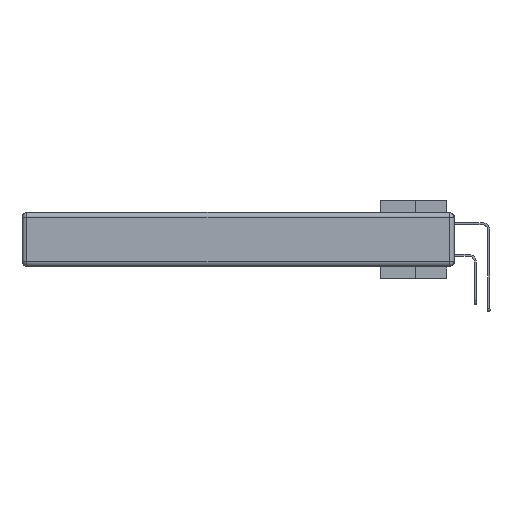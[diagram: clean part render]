
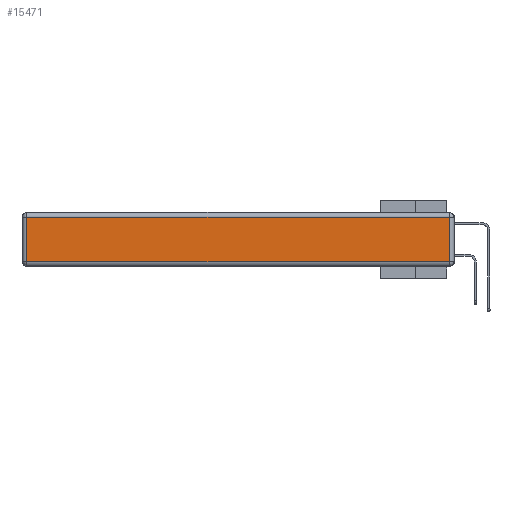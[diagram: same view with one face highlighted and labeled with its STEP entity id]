
A CAD part, left-side view. The second image highlights one B-rep face of the part: STEP entity #15471.
In plain terms, the highlighted planar face has unit normal (-1, 0, 0).
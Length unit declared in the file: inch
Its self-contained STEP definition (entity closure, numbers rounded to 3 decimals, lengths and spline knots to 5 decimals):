
#2451 = ORIENTED_EDGE ( 'NONE', *, *, #8380, .T. ) ;
#2903 = CARTESIAN_POINT ( 'NONE',  ( 0., 0., -0.313 ) ) ;
#3422 = VECTOR ( 'NONE', #16219, 39.37008 ) ;
#3586 = DIRECTION ( 'NONE',  ( 0., 0., -1. ) ) ;
#3810 = CARTESIAN_POINT ( 'NONE',  ( 0., 0., -0.343 ) ) ;
#4682 = VECTOR ( 'NONE', #9215, 39.37008 ) ;
#7297 = CARTESIAN_POINT ( 'NONE',  ( 0., 2.72, -0.343 ) ) ;
#7504 = CARTESIAN_POINT ( 'NONE',  ( 0., 0.03, -0.343 ) ) ;
#7738 = DIRECTION ( 'NONE',  ( 0., 0., 1. ) ) ;
#8380 = EDGE_CURVE ( 'NONE', #20937, #24700, #33931, .T. ) ;
#9215 = DIRECTION ( 'NONE',  ( 0., 1., 0. ) ) ;
#11574 = AXIS2_PLACEMENT_3D ( 'NONE', #3810, #40262, #7738 ) ;
#15471 = ADVANCED_FACE ( 'NONE', ( #26950 ), #40905, .T. ) ;
#16004 = ORIENTED_EDGE ( 'NONE', *, *, #37064, .T. ) ;
#16219 = DIRECTION ( 'NONE',  ( 0., -1., 0. ) ) ;
#16801 = VERTEX_POINT ( 'NONE', #38353 ) ;
#17663 = ORIENTED_EDGE ( 'NONE', *, *, #27846, .T. ) ;
#19945 = CARTESIAN_POINT ( 'NONE',  ( 0., 2.72, -0.313 ) ) ;
#20182 = LINE ( 'NONE', #7297, #41021 ) ;
#20229 = ORIENTED_EDGE ( 'NONE', *, *, #36000, .T. ) ;
#20713 = CARTESIAN_POINT ( 'NONE',  ( 0., 0.03, -0.313 ) ) ;
#20817 = DIRECTION ( 'NONE',  ( 0., 0., 1. ) ) ;
#20937 = VERTEX_POINT ( 'NONE', #20713 ) ;
#24700 = VERTEX_POINT ( 'NONE', #36340 ) ;
#25847 = LINE ( 'NONE', #38697, #4682 ) ;
#26950 = FACE_OUTER_BOUND ( 'NONE', #38497, .T. ) ;
#27846 = EDGE_CURVE ( 'NONE', #35707, #20937, #38936, .T. ) ;
#32406 = VECTOR ( 'NONE', #20817, 39.37008 ) ;
#33931 = LINE ( 'NONE', #7504, #32406 ) ;
#35707 = VERTEX_POINT ( 'NONE', #19945 ) ;
#36000 = EDGE_CURVE ( 'NONE', #24700, #16801, #25847, .T. ) ;
#36340 = CARTESIAN_POINT ( 'NONE',  ( 0., 0.03, -0.03 ) ) ;
#37064 = EDGE_CURVE ( 'NONE', #16801, #35707, #20182, .T. ) ;
#38353 = CARTESIAN_POINT ( 'NONE',  ( 0., 2.72, -0.03 ) ) ;
#38497 = EDGE_LOOP ( 'NONE', ( #17663, #2451, #20229, #16004 ) ) ;
#38697 = CARTESIAN_POINT ( 'NONE',  ( 0., 2.75, -0.03 ) ) ;
#38936 = LINE ( 'NONE', #2903, #3422 ) ;
#40262 = DIRECTION ( 'NONE',  ( -1., 0., 0. ) ) ;
#40905 = PLANE ( 'NONE',  #11574 ) ;
#41021 = VECTOR ( 'NONE', #3586, 39.37008 ) ;
